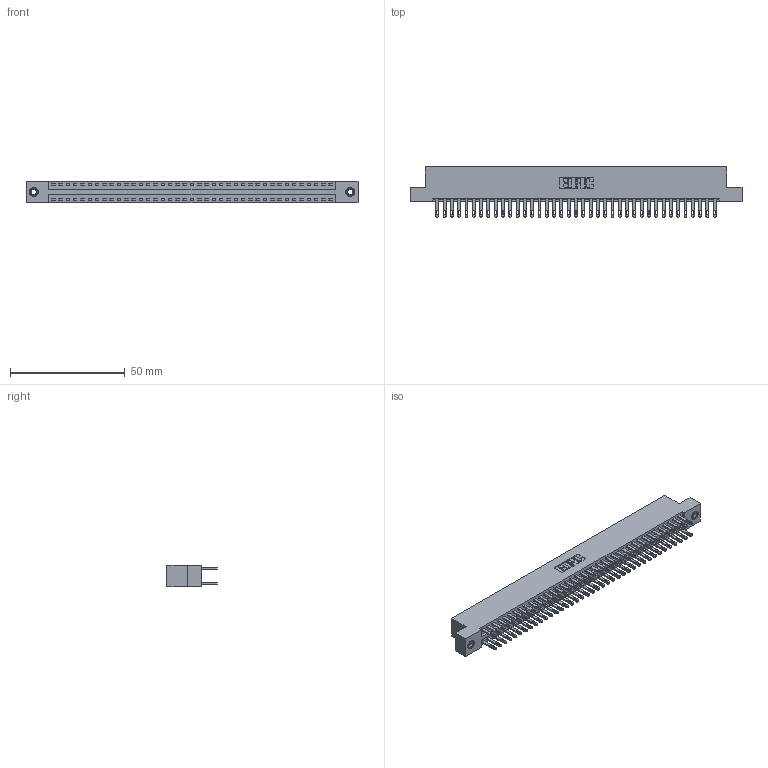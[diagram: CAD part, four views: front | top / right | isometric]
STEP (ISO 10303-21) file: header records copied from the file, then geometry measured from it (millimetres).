
FILE_DESCRIPTION (( 'STEP AP203' ), '1' );
FILE_NAME ('896-078-500-207.STEP', '2021-07-28T01:52:24', ( '' ), ( '' ), 'SwSTEP 2.0', 'SolidWorks 2020', '' );
FILE_SCHEMA (( 'CONFIG_CONTROL_DESIGN' ));
Length unit declared in the file: inch
Products named in the file (4): 345-250-001_345-250-005-103; 846 Part_Flush Mounting Lugs - 0.156 Dia-TI; 896-078-500-207; 345-292-001_345-293-100
Assembly tree (81 placements, depth 2):
  896-078-500-207
    846 Part_Flush Mounting Lugs - 0.156 Dia-TI
    345-292-001_345-293-100  x78
    345-250-001_345-250-005-103  x2
Bounding box: 144.4 x 21.84 x 9.4 mm (x, y, z)
Volume: 14282.2 mm3; surface area: 20434.9 mm2
Topology: 81 solids, 81 shells, 3926 faces, 11931 edges, 7946 vertices
Faces by surface type: plane 2370, cylinder 1540, cone 12, torus 4
Entity records: 26972 total; most frequent: CARTESIAN_POINT 4431, ORIENTED_EDGE 4358, DIRECTION 3985, EDGE_CURVE 2179, LINE 1867, VECTOR 1867, VERTEX_POINT 1448, AXIS2_PLACEMENT_3D 1059
